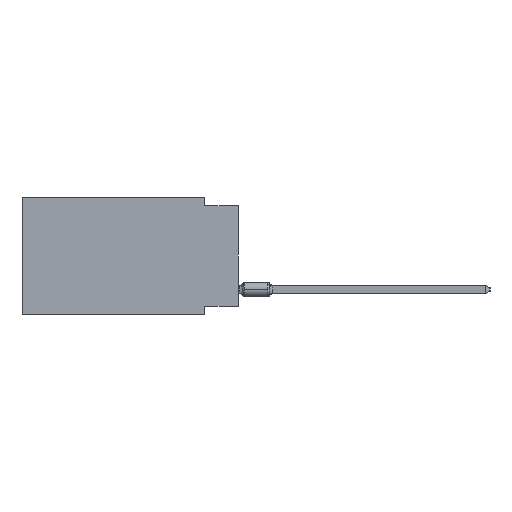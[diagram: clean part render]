
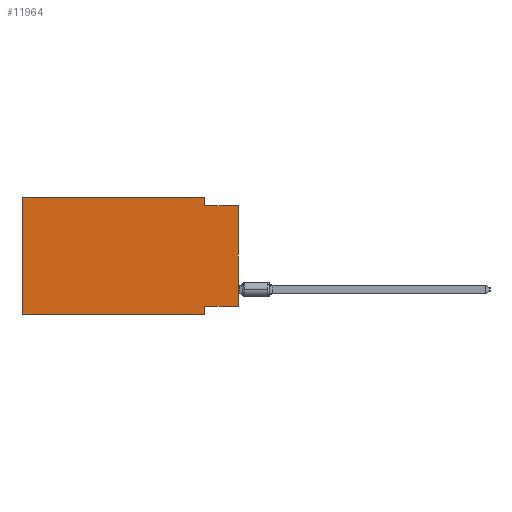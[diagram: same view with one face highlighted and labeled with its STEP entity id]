
A CAD part, left-side view. The second image highlights one B-rep face of the part: STEP entity #11964.
In plain terms, the highlighted planar face has unit normal (-1, 0, 0).
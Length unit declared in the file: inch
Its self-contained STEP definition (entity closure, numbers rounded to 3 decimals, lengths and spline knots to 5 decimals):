
#31 = CARTESIAN_POINT ( 'NONE',  ( 0., 0., -0.325 ) ) ;
#158 = DIRECTION ( 'NONE',  ( 0., 0., -1. ) ) ;
#345 = CARTESIAN_POINT ( 'NONE',  ( 0., 0.1, -0.025 ) ) ;
#576 = LINE ( 'NONE', #2667, #2475 ) ;
#1230 = CARTESIAN_POINT ( 'NONE',  ( 0., 0.645, 0. ) ) ;
#1468 = CARTESIAN_POINT ( 'NONE',  ( 0., 0., -0.325 ) ) ;
#1772 = ORIENTED_EDGE ( 'NONE', *, *, #15621, .F. ) ;
#2475 = VECTOR ( 'NONE', #22056, 39.37008 ) ;
#2582 = CARTESIAN_POINT ( 'NONE',  ( 0., 0., -0.025 ) ) ;
#2667 = CARTESIAN_POINT ( 'NONE',  ( 0., 0.645, 0. ) ) ;
#2964 = VECTOR ( 'NONE', #158, 39.37008 ) ;
#3685 = ORIENTED_EDGE ( 'NONE', *, *, #26192, .F. ) ;
#3962 = CARTESIAN_POINT ( 'NONE',  ( 0., 0.1, -0.325 ) ) ;
#4283 = ORIENTED_EDGE ( 'NONE', *, *, #24045, .F. ) ;
#4352 = CARTESIAN_POINT ( 'NONE',  ( 0., 0.1, 0. ) ) ;
#4362 = CARTESIAN_POINT ( 'NONE',  ( 0., 0., -0.025 ) ) ;
#6121 = LINE ( 'NONE', #27322, #2964 ) ;
#6184 = FACE_OUTER_BOUND ( 'NONE', #8811, .T. ) ;
#6429 = VERTEX_POINT ( 'NONE', #1468 ) ;
#6527 = VECTOR ( 'NONE', #21307, 39.37008 ) ;
#6748 = VECTOR ( 'NONE', #15491, 39.37008 ) ;
#6755 = CARTESIAN_POINT ( 'NONE',  ( 0., 0.645, 0. ) ) ;
#6783 = ORIENTED_EDGE ( 'NONE', *, *, #8459, .T. ) ;
#6890 = CARTESIAN_POINT ( 'NONE',  ( 0., 0.1, -0.35 ) ) ;
#8459 = EDGE_CURVE ( 'NONE', #6429, #23676, #17137, .T. ) ;
#8779 = VERTEX_POINT ( 'NONE', #4352 ) ;
#8811 = EDGE_LOOP ( 'NONE', ( #6783, #15512, #1772, #4283, #16023, #27116, #3685, #18157 ) ) ;
#8976 = LINE ( 'NONE', #6890, #6527 ) ;
#9278 = EDGE_CURVE ( 'NONE', #16753, #18265, #25738, .T. ) ;
#9977 = DIRECTION ( 'NONE',  ( 0., -1., 0. ) ) ;
#10349 = DIRECTION ( 'NONE',  ( 1., 0., 0. ) ) ;
#10478 = CARTESIAN_POINT ( 'NONE',  ( 0., 0.1, -0.35 ) ) ;
#11667 = LINE ( 'NONE', #22575, #21624 ) ;
#11964 = ADVANCED_FACE ( 'NONE', ( #6184 ), #12435, .F. ) ;
#12435 = PLANE ( 'NONE',  #17354 ) ;
#12784 = LINE ( 'NONE', #31, #25069 ) ;
#13672 = DIRECTION ( 'NONE',  ( 0., -1., 0. ) ) ;
#14784 = VERTEX_POINT ( 'NONE', #3962 ) ;
#14940 = VERTEX_POINT ( 'NONE', #10478 ) ;
#15491 = DIRECTION ( 'NONE',  ( 0., 0., 1. ) ) ;
#15512 = ORIENTED_EDGE ( 'NONE', *, *, #20985, .F. ) ;
#15621 = EDGE_CURVE ( 'NONE', #8779, #18910, #6121, .T. ) ;
#16023 = ORIENTED_EDGE ( 'NONE', *, *, #9278, .F. ) ;
#16360 = CARTESIAN_POINT ( 'NONE',  ( 0., 0., 0. ) ) ;
#16753 = VERTEX_POINT ( 'NONE', #26045 ) ;
#17137 = LINE ( 'NONE', #16360, #24539 ) ;
#17354 = AXIS2_PLACEMENT_3D ( 'NONE', #20869, #10349, #18779 ) ;
#18157 = ORIENTED_EDGE ( 'NONE', *, *, #22804, .F. ) ;
#18265 = VERTEX_POINT ( 'NONE', #1230 ) ;
#18779 = DIRECTION ( 'NONE',  ( 0., 0., -1. ) ) ;
#18910 = VERTEX_POINT ( 'NONE', #345 ) ;
#19870 = LINE ( 'NONE', #2582, #26364 ) ;
#20364 = DIRECTION ( 'NONE',  ( 0., 0., 1. ) ) ;
#20814 = DIRECTION ( 'NONE',  ( 0., 1., 0. ) ) ;
#20869 = CARTESIAN_POINT ( 'NONE',  ( 0., 0.645, 0. ) ) ;
#20985 = EDGE_CURVE ( 'NONE', #18910, #23676, #19870, .T. ) ;
#21307 = DIRECTION ( 'NONE',  ( 0., 0., -1. ) ) ;
#21624 = VECTOR ( 'NONE', #9977, 39.37008 ) ;
#22056 = DIRECTION ( 'NONE',  ( 0., -1., 0. ) ) ;
#22575 = CARTESIAN_POINT ( 'NONE',  ( 0., 0.645, -0.35 ) ) ;
#22804 = EDGE_CURVE ( 'NONE', #6429, #14784, #12784, .T. ) ;
#23676 = VERTEX_POINT ( 'NONE', #4362 ) ;
#24045 = EDGE_CURVE ( 'NONE', #18265, #8779, #576, .T. ) ;
#24539 = VECTOR ( 'NONE', #20364, 39.37008 ) ;
#25069 = VECTOR ( 'NONE', #20814, 39.37008 ) ;
#25738 = LINE ( 'NONE', #6755, #6748 ) ;
#26045 = CARTESIAN_POINT ( 'NONE',  ( 0., 0.645, -0.35 ) ) ;
#26192 = EDGE_CURVE ( 'NONE', #14784, #14940, #8976, .T. ) ;
#26364 = VECTOR ( 'NONE', #13672, 39.37008 ) ;
#27116 = ORIENTED_EDGE ( 'NONE', *, *, #27179, .T. ) ;
#27179 = EDGE_CURVE ( 'NONE', #16753, #14940, #11667, .T. ) ;
#27322 = CARTESIAN_POINT ( 'NONE',  ( 0., 0.1, 0. ) ) ;
